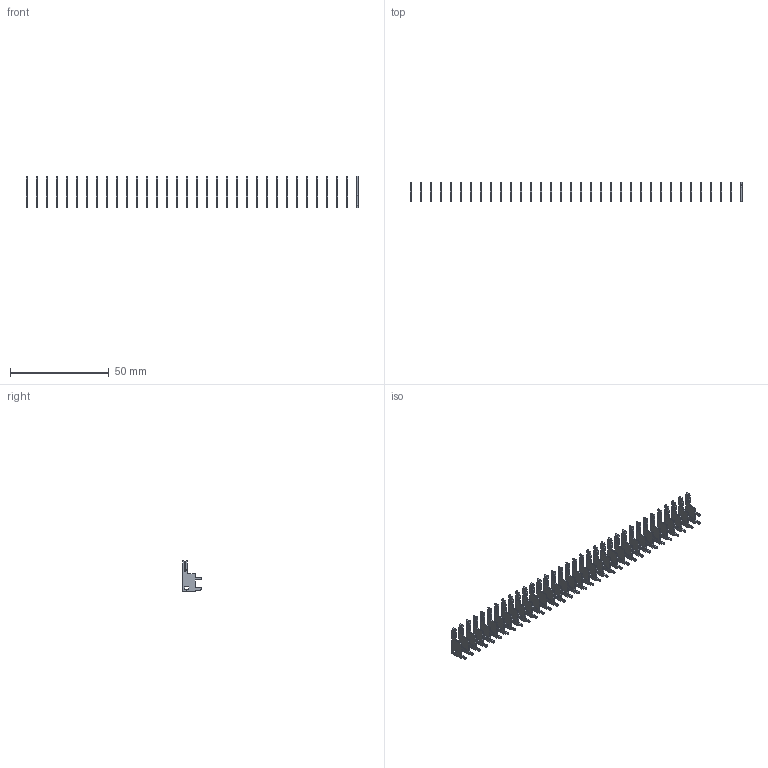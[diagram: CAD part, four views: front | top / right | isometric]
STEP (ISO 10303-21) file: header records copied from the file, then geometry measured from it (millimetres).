
FILE_DESCRIPTION (( 'STEP AP203' ), '1' );
FILE_NAME ('105-034-201-200.STEP', '2020-04-07T23:37:22', ( '' ), ( '' ), 'SwSTEP 2.0', 'SolidWorks 2016', '' );
FILE_SCHEMA (( 'CONFIG_CONTROL_DESIGN' ));
Length unit declared in the file: inch
Products named in the file (2): 100-290-001_100-290-201; 105-034-201-200
Assembly tree (34 placements, depth 2):
  105-034-201-200
    100-290-001_100-290-201  x34
Bounding box: 168.28 x 9.7 x 15.88 mm (x, y, z)
Volume: 1674.2 mm3; surface area: 6832 mm2
Topology: 34 solids, 34 shells, 1190 faces, 3366 edges, 2244 vertices
Faces by surface type: plane 850, cylinder 340
Entity records: 2393 total; most frequent: DIRECTION 259, CARTESIAN_POINT 249, ORIENTED_EDGE 198, EDGE_CURVE 99, AXIS2_PLACEMENT_3D 92, LOCAL_TIME 78, DATE_AND_TIME 78, COORDINATED_UNIVERSAL_TIME_OFFSET 78
